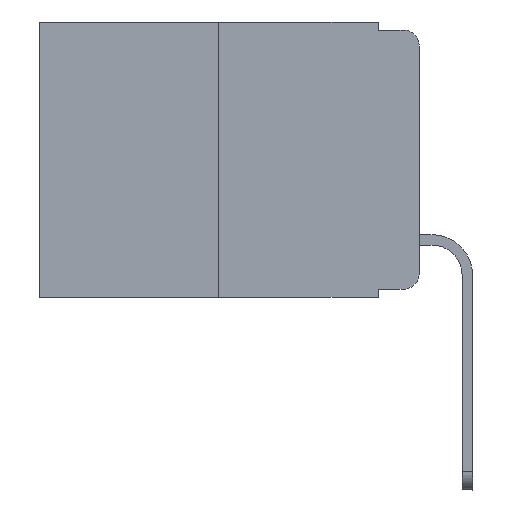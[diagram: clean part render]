
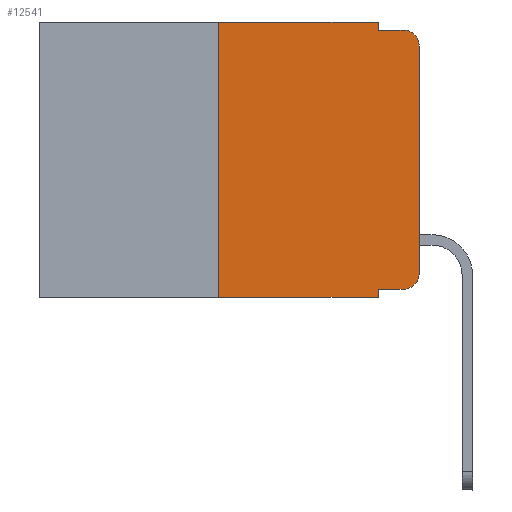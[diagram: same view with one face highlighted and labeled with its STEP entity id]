
A CAD part, left-side view. The second image highlights one B-rep face of the part: STEP entity #12541.
In plain terms, the highlighted planar face has unit normal (-1, 0, 0).
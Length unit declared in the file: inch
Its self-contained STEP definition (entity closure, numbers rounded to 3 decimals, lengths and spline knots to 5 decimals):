
#227 = EDGE_CURVE ( 'NONE', #14045, #4528, #1314, .T. ) ;
#289 = CARTESIAN_POINT ( 'NONE',  ( 0., 0., 0. ) ) ;
#335 = DIRECTION ( 'NONE',  ( 0., -1., 0. ) ) ;
#468 = CARTESIAN_POINT ( 'NONE',  ( 0., 0.051, -0.01 ) ) ;
#501 = ORIENTED_EDGE ( 'NONE', *, *, #7613, .T. ) ;
#590 = VECTOR ( 'NONE', #1088, 39.37008 ) ;
#973 = EDGE_CURVE ( 'NONE', #3008, #12589, #4465, .T. ) ;
#1088 = DIRECTION ( 'NONE',  ( 0., -1., 0. ) ) ;
#1314 = LINE ( 'NONE', #289, #2940 ) ;
#1528 = CARTESIAN_POINT ( 'NONE',  ( 0., 0., -0.03 ) ) ;
#1904 = EDGE_CURVE ( 'NONE', #12589, #1929, #2723, .T. ) ;
#1929 = VERTEX_POINT ( 'NONE', #6772 ) ;
#1946 = EDGE_CURVE ( 'NONE', #9141, #3008, #9044, .T. ) ;
#1967 = VERTEX_POINT ( 'NONE', #9910 ) ;
#2088 = DIRECTION ( 'NONE',  ( 0., 0., -1. ) ) ;
#2126 = VECTOR ( 'NONE', #13533, 39.37008 ) ;
#2391 = DIRECTION ( 'NONE',  ( 0., 0., 1. ) ) ;
#2404 = CARTESIAN_POINT ( 'NONE',  ( 0., 0.473, 0. ) ) ;
#2478 = VERTEX_POINT ( 'NONE', #6826 ) ;
#2723 = LINE ( 'NONE', #11230, #12776 ) ;
#2899 = VERTEX_POINT ( 'NONE', #8858 ) ;
#2940 = VECTOR ( 'NONE', #11253, 39.37008 ) ;
#3008 = VERTEX_POINT ( 'NONE', #9148 ) ;
#3421 = EDGE_CURVE ( 'NONE', #1967, #11704, #9269, .T. ) ;
#3451 = ORIENTED_EDGE ( 'NONE', *, *, #973, .F. ) ;
#3636 = DIRECTION ( 'NONE',  ( 1., 0., 0. ) ) ;
#3795 = AXIS2_PLACEMENT_3D ( 'NONE', #9164, #5631, #6895 ) ;
#4465 = LINE ( 'NONE', #9027, #13756 ) ;
#4528 = VERTEX_POINT ( 'NONE', #1528 ) ;
#4550 = LINE ( 'NONE', #12395, #8548 ) ;
#4761 = CARTESIAN_POINT ( 'NONE',  ( 0., 0.051, -0.333 ) ) ;
#5240 = ORIENTED_EDGE ( 'NONE', *, *, #3421, .F. ) ;
#5447 = ORIENTED_EDGE ( 'NONE', *, *, #1904, .F. ) ;
#5631 = DIRECTION ( 'NONE',  ( -1., 0., 0. ) ) ;
#5960 = CARTESIAN_POINT ( 'NONE',  ( 0., 0., -0.313 ) ) ;
#6068 = VECTOR ( 'NONE', #335, 39.37008 ) ;
#6607 = DIRECTION ( 'NONE',  ( -1., 0., 0. ) ) ;
#6772 = CARTESIAN_POINT ( 'NONE',  ( 0., 0.02, -0.01 ) ) ;
#6826 = CARTESIAN_POINT ( 'NONE',  ( 0., 0.25, -0.343 ) ) ;
#6895 = DIRECTION ( 'NONE',  ( 0., 0., -1. ) ) ;
#6974 = DIRECTION ( 'NONE',  ( 0., -1., 0. ) ) ;
#7110 = CIRCLE ( 'NONE', #3795, 0.02 ) ;
#7116 = LINE ( 'NONE', #10414, #6068 ) ;
#7365 = EDGE_CURVE ( 'NONE', #2478, #11704, #7116, .T. ) ;
#7613 = EDGE_CURVE ( 'NONE', #4528, #1929, #9586, .T. ) ;
#7799 = DIRECTION ( 'NONE',  ( 0., -1., 0. ) ) ;
#7864 = FACE_OUTER_BOUND ( 'NONE', #9476, .T. ) ;
#7912 = ORIENTED_EDGE ( 'NONE', *, *, #227, .T. ) ;
#7937 = CARTESIAN_POINT ( 'NONE',  ( 0., 0.25, 0. ) ) ;
#8076 = DIRECTION ( 'NONE',  ( 0., 0., -1. ) ) ;
#8276 = AXIS2_PLACEMENT_3D ( 'NONE', #13715, #3636, #13503 ) ;
#8548 = VECTOR ( 'NONE', #2391, 39.37008 ) ;
#8858 = CARTESIAN_POINT ( 'NONE',  ( 0., 0.02, -0.333 ) ) ;
#9027 = CARTESIAN_POINT ( 'NONE',  ( 0., 0.051, 0. ) ) ;
#9030 = VECTOR ( 'NONE', #6974, 39.37008 ) ;
#9044 = LINE ( 'NONE', #2404, #590 ) ;
#9141 = VERTEX_POINT ( 'NONE', #7937 ) ;
#9148 = CARTESIAN_POINT ( 'NONE',  ( 0., 0.051, 0. ) ) ;
#9164 = CARTESIAN_POINT ( 'NONE',  ( 0., 0.02, -0.313 ) ) ;
#9269 = LINE ( 'NONE', #13742, #2126 ) ;
#9476 = EDGE_LOOP ( 'NONE', ( #7912, #501, #5447, #3451, #11377, #10891, #9571, #5240, #9820, #10221 ) ) ;
#9571 = ORIENTED_EDGE ( 'NONE', *, *, #7365, .T. ) ;
#9586 = CIRCLE ( 'NONE', #11462, 0.02 ) ;
#9820 = ORIENTED_EDGE ( 'NONE', *, *, #14419, .T. ) ;
#9910 = CARTESIAN_POINT ( 'NONE',  ( 0., 0.051, -0.333 ) ) ;
#10221 = ORIENTED_EDGE ( 'NONE', *, *, #12889, .T. ) ;
#10242 = CARTESIAN_POINT ( 'NONE',  ( 0., 0.051, -0.343 ) ) ;
#10414 = CARTESIAN_POINT ( 'NONE',  ( 0., 0.473, -0.343 ) ) ;
#10891 = ORIENTED_EDGE ( 'NONE', *, *, #14512, .F. ) ;
#11230 = CARTESIAN_POINT ( 'NONE',  ( 0., 0.051, -0.01 ) ) ;
#11253 = DIRECTION ( 'NONE',  ( 0., 0., 1. ) ) ;
#11377 = ORIENTED_EDGE ( 'NONE', *, *, #1946, .F. ) ;
#11462 = AXIS2_PLACEMENT_3D ( 'NONE', #13121, #6607, #2088 ) ;
#11704 = VERTEX_POINT ( 'NONE', #10242 ) ;
#12395 = CARTESIAN_POINT ( 'NONE',  ( 0., 0.25, 0. ) ) ;
#12541 = ADVANCED_FACE ( 'NONE', ( #7864 ), #12595, .F. ) ;
#12589 = VERTEX_POINT ( 'NONE', #468 ) ;
#12593 = LINE ( 'NONE', #4761, #9030 ) ;
#12595 = PLANE ( 'NONE',  #8276 ) ;
#12776 = VECTOR ( 'NONE', #7799, 39.37008 ) ;
#12889 = EDGE_CURVE ( 'NONE', #2899, #14045, #7110, .T. ) ;
#13121 = CARTESIAN_POINT ( 'NONE',  ( 0., 0.02, -0.03 ) ) ;
#13503 = DIRECTION ( 'NONE',  ( 0., 0., -1. ) ) ;
#13533 = DIRECTION ( 'NONE',  ( 0., 0., -1. ) ) ;
#13715 = CARTESIAN_POINT ( 'NONE',  ( 0., 0.473, 0. ) ) ;
#13742 = CARTESIAN_POINT ( 'NONE',  ( 0., 0.051, 0. ) ) ;
#13756 = VECTOR ( 'NONE', #8076, 39.37008 ) ;
#14045 = VERTEX_POINT ( 'NONE', #5960 ) ;
#14419 = EDGE_CURVE ( 'NONE', #1967, #2899, #12593, .T. ) ;
#14512 = EDGE_CURVE ( 'NONE', #2478, #9141, #4550, .T. ) ;
